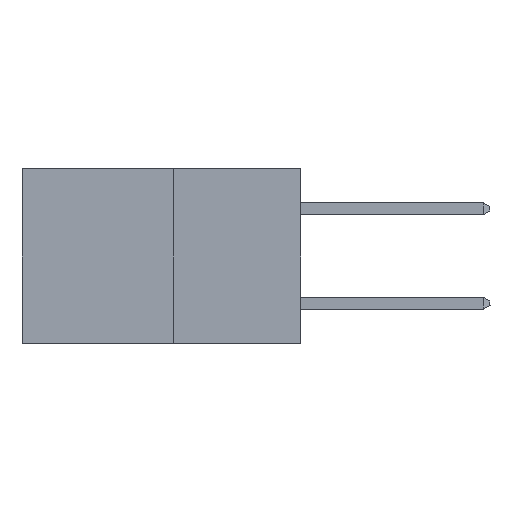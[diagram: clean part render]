
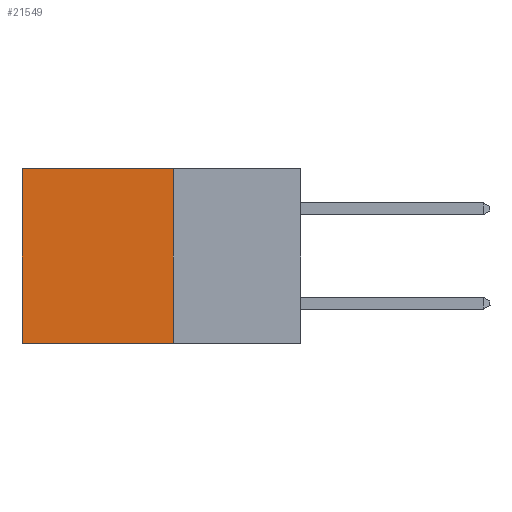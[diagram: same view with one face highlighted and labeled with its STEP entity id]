
A CAD part, left-side view. The second image highlights one B-rep face of the part: STEP entity #21549.
In plain terms, the highlighted planar face has unit normal (-1, 0, 0).
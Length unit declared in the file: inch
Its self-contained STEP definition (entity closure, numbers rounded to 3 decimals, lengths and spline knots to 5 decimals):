
#1931 = ORIENTED_EDGE ( 'NONE', *, *, #10196, .T. ) ;
#2071 = DIRECTION ( 'NONE',  ( 0., 0., -1. ) ) ;
#2285 = VERTEX_POINT ( 'NONE', #10112 ) ;
#2430 = CARTESIAN_POINT ( 'NONE',  ( 0.277, 0.27, 0. ) ) ;
#2947 = CARTESIAN_POINT ( 'NONE',  ( 0.277, 0.27, -0.37 ) ) ;
#3516 = LINE ( 'NONE', #2947, #12262 ) ;
#6555 = ORIENTED_EDGE ( 'NONE', *, *, #14795, .F. ) ;
#6725 = VECTOR ( 'NONE', #15449, 39.37008 ) ;
#7104 = CARTESIAN_POINT ( 'NONE',  ( 0.277, 0.27, -0.37 ) ) ;
#7222 = AXIS2_PLACEMENT_3D ( 'NONE', #13360, #20757, #9746 ) ;
#8856 = ORIENTED_EDGE ( 'NONE', *, *, #18480, .T. ) ;
#8971 = DIRECTION ( 'NONE',  ( 0., 1., 0. ) ) ;
#9704 = EDGE_CURVE ( 'NONE', #9881, #23748, #3516, .T. ) ;
#9746 = DIRECTION ( 'NONE',  ( 0., 0., -1. ) ) ;
#9881 = VERTEX_POINT ( 'NONE', #14478 ) ;
#10112 = CARTESIAN_POINT ( 'NONE',  ( 0.277, 0.59, -0.37 ) ) ;
#10196 = EDGE_CURVE ( 'NONE', #9881, #10496, #11075, .T. ) ;
#10496 = VERTEX_POINT ( 'NONE', #18164 ) ;
#11075 = LINE ( 'NONE', #2430, #6725 ) ;
#11425 = EDGE_LOOP ( 'NONE', ( #8856, #6555, #16082, #1931 ) ) ;
#12262 = VECTOR ( 'NONE', #17759, 39.37008 ) ;
#13360 = CARTESIAN_POINT ( 'NONE',  ( 0.277, 0.27, -0.37 ) ) ;
#14478 = CARTESIAN_POINT ( 'NONE',  ( 0.277, 0.27, 0. ) ) ;
#14650 = LINE ( 'NONE', #7104, #23806 ) ;
#14795 = EDGE_CURVE ( 'NONE', #23748, #2285, #14650, .T. ) ;
#15449 = DIRECTION ( 'NONE',  ( 0., 1., 0. ) ) ;
#16082 = ORIENTED_EDGE ( 'NONE', *, *, #9704, .F. ) ;
#16760 = LINE ( 'NONE', #20556, #21105 ) ;
#17759 = DIRECTION ( 'NONE',  ( 0., 0., -1. ) ) ;
#18164 = CARTESIAN_POINT ( 'NONE',  ( 0.277, 0.59, 0. ) ) ;
#18480 = EDGE_CURVE ( 'NONE', #10496, #2285, #16760, .T. ) ;
#18897 = PLANE ( 'NONE',  #7222 ) ;
#20556 = CARTESIAN_POINT ( 'NONE',  ( 0.277, 0.59, -0.37 ) ) ;
#20757 = DIRECTION ( 'NONE',  ( 1., 0., 0. ) ) ;
#20990 = CARTESIAN_POINT ( 'NONE',  ( 0.277, 0.27, -0.37 ) ) ;
#21105 = VECTOR ( 'NONE', #2071, 39.37008 ) ;
#21140 = FACE_OUTER_BOUND ( 'NONE', #11425, .T. ) ;
#21549 = ADVANCED_FACE ( 'NONE', ( #21140 ), #18897, .F. ) ;
#23748 = VERTEX_POINT ( 'NONE', #20990 ) ;
#23806 = VECTOR ( 'NONE', #8971, 39.37008 ) ;
